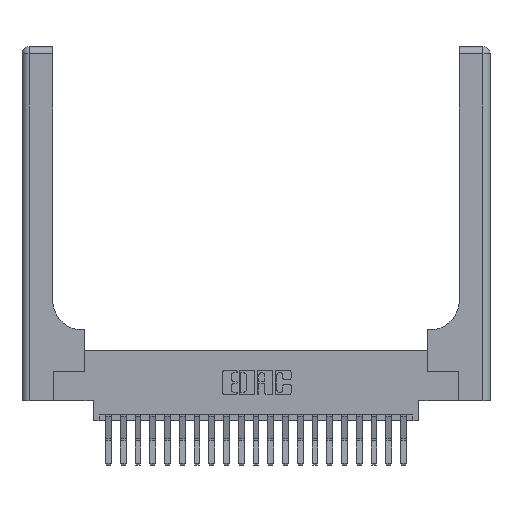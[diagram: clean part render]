
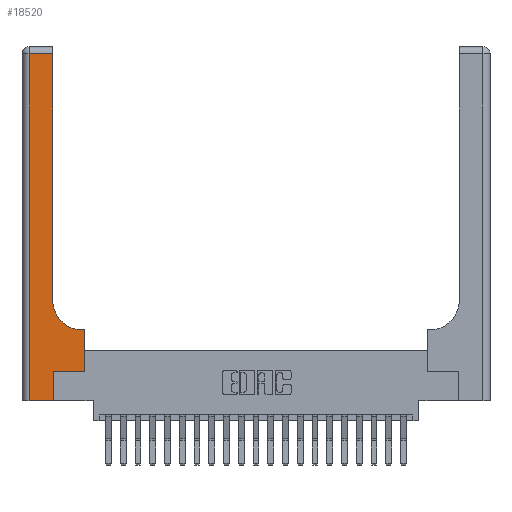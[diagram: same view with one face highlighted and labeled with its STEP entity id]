
A CAD part, top view. The second image highlights one B-rep face of the part: STEP entity #18520.
In plain terms, the highlighted planar face has unit normal (0, 0, 1).
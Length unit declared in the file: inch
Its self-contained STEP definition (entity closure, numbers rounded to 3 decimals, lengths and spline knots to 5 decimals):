
#1110 = DIRECTION ( 'NONE',  ( -1., 0., 0. ) ) ;
#1204 = DIRECTION ( 'NONE',  ( -1., 0., 0. ) ) ;
#1711 = CARTESIAN_POINT ( 'NONE',  ( 0.265, 0., 0.37 ) ) ;
#1759 = VERTEX_POINT ( 'NONE', #13410 ) ;
#2675 = CARTESIAN_POINT ( 'NONE',  ( 0.26, 0.85, 0.37 ) ) ;
#2868 = EDGE_CURVE ( 'NONE', #18493, #21836, #3893, .T. ) ;
#2899 = CARTESIAN_POINT ( 'NONE',  ( 0.26, 0.6, 0.37 ) ) ;
#3085 = LINE ( 'NONE', #1711, #7142 ) ;
#3327 = VECTOR ( 'NONE', #1110, 39.37008 ) ;
#3496 = CARTESIAN_POINT ( 'NONE',  ( 0.528, 0.25, 0.37 ) ) ;
#3893 = LINE ( 'NONE', #12462, #16102 ) ;
#3965 = DIRECTION ( 'NONE',  ( 0., -1., 0. ) ) ;
#4350 = EDGE_CURVE ( 'NONE', #9612, #8399, #12348, .T. ) ;
#4614 = LINE ( 'NONE', #2899, #8950 ) ;
#5693 = LINE ( 'NONE', #12532, #16494 ) ;
#5742 = VERTEX_POINT ( 'NONE', #8284 ) ;
#6130 = DIRECTION ( 'NONE',  ( 0., 0., -1. ) ) ;
#6403 = CARTESIAN_POINT ( 'NONE',  ( 0.265, 0., 0.37 ) ) ;
#6492 = EDGE_LOOP ( 'NONE', ( #11384, #12581, #14265, #6747, #19748, #12206, #17421, #6544, #17520 ) ) ;
#6544 = ORIENTED_EDGE ( 'NONE', *, *, #15742, .T. ) ;
#6673 = VERTEX_POINT ( 'NONE', #17368 ) ;
#6747 = ORIENTED_EDGE ( 'NONE', *, *, #11174, .T. ) ;
#7142 = VECTOR ( 'NONE', #15146, 39.37008 ) ;
#7156 = VERTEX_POINT ( 'NONE', #6403 ) ;
#7237 = FACE_OUTER_BOUND ( 'NONE', #6492, .T. ) ;
#7363 = EDGE_CURVE ( 'NONE', #7156, #18493, #3085, .T. ) ;
#7835 = CARTESIAN_POINT ( 'NONE',  ( 0.528, 0.6, 0.37 ) ) ;
#7907 = DIRECTION ( 'NONE',  ( 1., 0., 0. ) ) ;
#7910 = CARTESIAN_POINT ( 'NONE',  ( 0.528, 0.25, 0.37 ) ) ;
#8284 = CARTESIAN_POINT ( 'NONE',  ( 0.06, 2.94, 0.37 ) ) ;
#8399 = VERTEX_POINT ( 'NONE', #15986 ) ;
#8950 = VECTOR ( 'NONE', #1204, 39.37008 ) ;
#9094 = DIRECTION ( 'NONE',  ( 0., 1., 0. ) ) ;
#9612 = VERTEX_POINT ( 'NONE', #2675 ) ;
#10009 = CARTESIAN_POINT ( 'NONE',  ( 0., 2.94, 0.37 ) ) ;
#10321 = LINE ( 'NONE', #12127, #12054 ) ;
#10353 = CARTESIAN_POINT ( 'NONE',  ( 0., 3., 0.37 ) ) ;
#10758 = DIRECTION ( 'NONE',  ( 1., 0., 0. ) ) ;
#10807 = PLANE ( 'NONE',  #21328 ) ;
#11174 = EDGE_CURVE ( 'NONE', #1759, #7156, #10321, .T. ) ;
#11384 = ORIENTED_EDGE ( 'NONE', *, *, #4350, .T. ) ;
#11961 = CIRCLE ( 'NONE', #15188, 0.25 ) ;
#12054 = VECTOR ( 'NONE', #13924, 39.37008 ) ;
#12127 = CARTESIAN_POINT ( 'NONE',  ( 0., 0., 0.37 ) ) ;
#12206 = ORIENTED_EDGE ( 'NONE', *, *, #2868, .T. ) ;
#12348 = LINE ( 'NONE', #21078, #15786 ) ;
#12393 = CARTESIAN_POINT ( 'NONE',  ( 0.265, 0.25, 0.37 ) ) ;
#12462 = CARTESIAN_POINT ( 'NONE',  ( 0.265, 0.25, 0.37 ) ) ;
#12532 = CARTESIAN_POINT ( 'NONE',  ( 0.06, 3., 0.37 ) ) ;
#12581 = ORIENTED_EDGE ( 'NONE', *, *, #20868, .T. ) ;
#12848 = CARTESIAN_POINT ( 'NONE',  ( 0.51, 0.85, 0.37 ) ) ;
#13356 = EDGE_CURVE ( 'NONE', #5742, #1759, #5693, .T. ) ;
#13410 = CARTESIAN_POINT ( 'NONE',  ( 0.06, 0., 0.37 ) ) ;
#13924 = DIRECTION ( 'NONE',  ( 1., 0., 0. ) ) ;
#14100 = VECTOR ( 'NONE', #16118, 39.37008 ) ;
#14197 = DIRECTION ( 'NONE',  ( 0., 0., -1. ) ) ;
#14265 = ORIENTED_EDGE ( 'NONE', *, *, #13356, .T. ) ;
#15146 = DIRECTION ( 'NONE',  ( 0., 1., 0. ) ) ;
#15188 = AXIS2_PLACEMENT_3D ( 'NONE', #12848, #6130, #7907 ) ;
#15742 = EDGE_CURVE ( 'NONE', #21610, #6673, #4614, .T. ) ;
#15786 = VECTOR ( 'NONE', #9094, 39.37008 ) ;
#15986 = CARTESIAN_POINT ( 'NONE',  ( 0.26, 2.94, 0.37 ) ) ;
#16102 = VECTOR ( 'NONE', #10758, 39.37008 ) ;
#16118 = DIRECTION ( 'NONE',  ( 0., 1., 0. ) ) ;
#16494 = VECTOR ( 'NONE', #3965, 39.37008 ) ;
#17368 = CARTESIAN_POINT ( 'NONE',  ( 0.51, 0.6, 0.37 ) ) ;
#17421 = ORIENTED_EDGE ( 'NONE', *, *, #22033, .T. ) ;
#17520 = ORIENTED_EDGE ( 'NONE', *, *, #20798, .T. ) ;
#18493 = VERTEX_POINT ( 'NONE', #12393 ) ;
#18520 = ADVANCED_FACE ( 'NONE', ( #7237 ), #10807, .F. ) ;
#19193 = DIRECTION ( 'NONE',  ( -1., 0., 0. ) ) ;
#19748 = ORIENTED_EDGE ( 'NONE', *, *, #7363, .T. ) ;
#20334 = LINE ( 'NONE', #10009, #3327 ) ;
#20798 = EDGE_CURVE ( 'NONE', #6673, #9612, #11961, .T. ) ;
#20868 = EDGE_CURVE ( 'NONE', #8399, #5742, #20334, .T. ) ;
#21078 = CARTESIAN_POINT ( 'NONE',  ( 0.26, 3., 0.37 ) ) ;
#21328 = AXIS2_PLACEMENT_3D ( 'NONE', #10353, #14197, #19193 ) ;
#21593 = LINE ( 'NONE', #7910, #14100 ) ;
#21610 = VERTEX_POINT ( 'NONE', #7835 ) ;
#21836 = VERTEX_POINT ( 'NONE', #3496 ) ;
#22033 = EDGE_CURVE ( 'NONE', #21836, #21610, #21593, .T. ) ;
